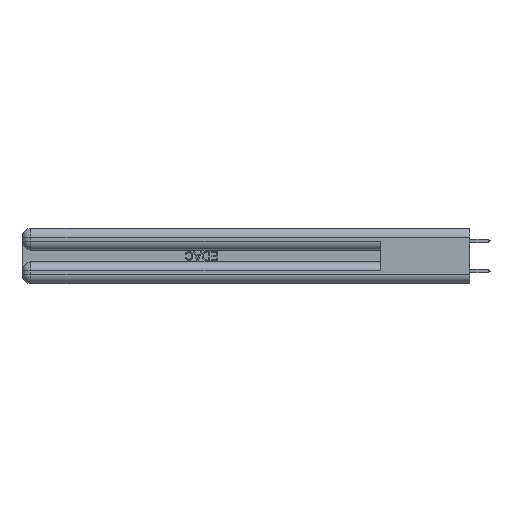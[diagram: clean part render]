
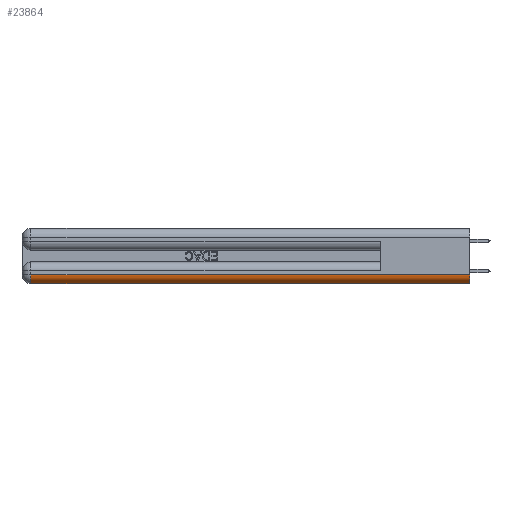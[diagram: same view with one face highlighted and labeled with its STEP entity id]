
A CAD part, left-side view. The second image highlights one B-rep face of the part: STEP entity #23864.
In plain terms, the highlighted cylindrical face has radius 1.524 mm (diameter 3.048 mm), a partial arc.
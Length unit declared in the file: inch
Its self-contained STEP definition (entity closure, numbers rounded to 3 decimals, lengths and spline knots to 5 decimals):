
#221 = VECTOR ( 'NONE', #22437, 39.37008 ) ;
#981 = DIRECTION ( 'NONE',  ( 0., 1., 0. ) ) ;
#2512 = DIRECTION ( 'NONE',  ( 0., -1., 0. ) ) ;
#3537 = DIRECTION ( 'NONE',  ( 0., 0., 1. ) ) ;
#3722 = CARTESIAN_POINT ( 'NONE',  ( 0.06, 2.94, 0. ) ) ;
#5727 = CIRCLE ( 'NONE', #36041, 0.06 ) ;
#5790 = DIRECTION ( 'NONE',  ( 0., 0., 1. ) ) ;
#6708 = VERTEX_POINT ( 'NONE', #35683 ) ;
#6767 = EDGE_LOOP ( 'NONE', ( #13103, #19667, #35469, #32025 ) ) ;
#8678 = LINE ( 'NONE', #32856, #28439 ) ;
#11909 = AXIS2_PLACEMENT_3D ( 'NONE', #32315, #38682, #3537 ) ;
#13103 = ORIENTED_EDGE ( 'NONE', *, *, #34833, .F. ) ;
#13979 = CARTESIAN_POINT ( 'NONE',  ( 0.06, 2.94, 0.06 ) ) ;
#18742 = CYLINDRICAL_SURFACE ( 'NONE', #11909, 0.06 ) ;
#19459 = CARTESIAN_POINT ( 'NONE',  ( 0., 0., 0.06 ) ) ;
#19667 = ORIENTED_EDGE ( 'NONE', *, *, #25619, .F. ) ;
#19969 = VERTEX_POINT ( 'NONE', #19459 ) ;
#20551 = CARTESIAN_POINT ( 'NONE',  ( 0., 2.94, 0.06 ) ) ;
#22437 = DIRECTION ( 'NONE',  ( 0., -1., 0. ) ) ;
#23192 = VERTEX_POINT ( 'NONE', #3722 ) ;
#23339 = DIRECTION ( 'NONE',  ( 0., 0., 1. ) ) ;
#23864 = ADVANCED_FACE ( 'NONE', ( #28899 ), #18742, .T. ) ;
#23907 = AXIS2_PLACEMENT_3D ( 'NONE', #37954, #2512, #5790 ) ;
#24058 = VERTEX_POINT ( 'NONE', #20551 ) ;
#25619 = EDGE_CURVE ( 'NONE', #24058, #19969, #33758, .T. ) ;
#25984 = CARTESIAN_POINT ( 'NONE',  ( 0., 0., 0.06 ) ) ;
#27812 = EDGE_CURVE ( 'NONE', #6708, #23192, #8678, .T. ) ;
#28439 = VECTOR ( 'NONE', #41801, 39.37008 ) ;
#28899 = FACE_OUTER_BOUND ( 'NONE', #6767, .T. ) ;
#32025 = ORIENTED_EDGE ( 'NONE', *, *, #27812, .F. ) ;
#32315 = CARTESIAN_POINT ( 'NONE',  ( 0.06, 0., 0.06 ) ) ;
#32323 = CIRCLE ( 'NONE', #23907, 0.06 ) ;
#32856 = CARTESIAN_POINT ( 'NONE',  ( 0.06, 3., 0. ) ) ;
#32857 = EDGE_CURVE ( 'NONE', #23192, #24058, #5727, .T. ) ;
#33758 = LINE ( 'NONE', #25984, #221 ) ;
#34833 = EDGE_CURVE ( 'NONE', #19969, #6708, #32323, .T. ) ;
#35469 = ORIENTED_EDGE ( 'NONE', *, *, #32857, .F. ) ;
#35683 = CARTESIAN_POINT ( 'NONE',  ( 0.06, 0., 0. ) ) ;
#36041 = AXIS2_PLACEMENT_3D ( 'NONE', #13979, #981, #23339 ) ;
#37954 = CARTESIAN_POINT ( 'NONE',  ( 0.06, 0., 0.06 ) ) ;
#38682 = DIRECTION ( 'NONE',  ( 0., 1., 0. ) ) ;
#41801 = DIRECTION ( 'NONE',  ( 0., 1., 0. ) ) ;
